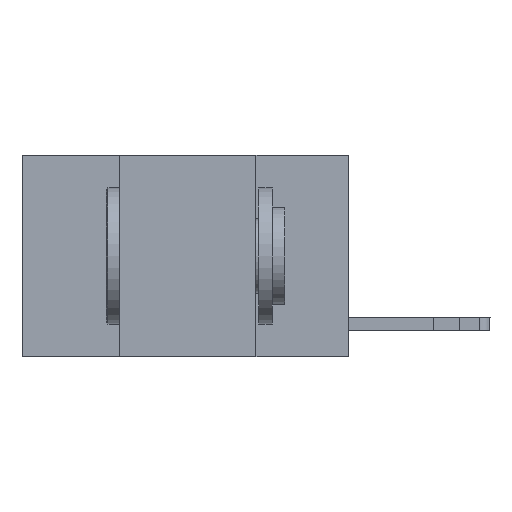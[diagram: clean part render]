
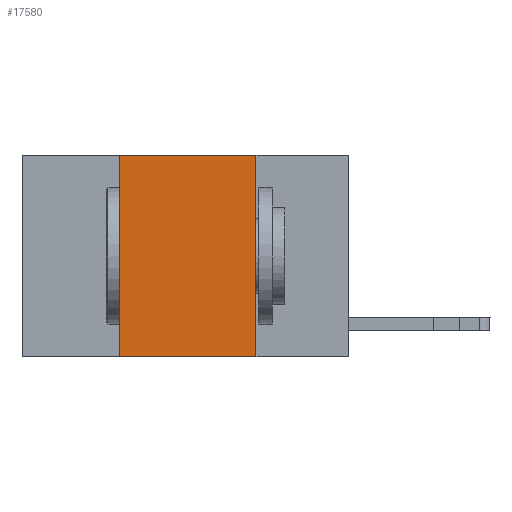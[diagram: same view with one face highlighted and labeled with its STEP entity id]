
A CAD part, left-side view. The second image highlights one B-rep face of the part: STEP entity #17580.
In plain terms, the highlighted planar face has unit normal (-1, 0, 0).
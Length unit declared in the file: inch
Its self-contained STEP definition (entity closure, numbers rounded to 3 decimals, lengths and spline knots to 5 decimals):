
#30 = VECTOR ( 'NONE', #4985, 39.37008 ) ;
#475 = EDGE_CURVE ( 'NONE', #6820, #13856, #2830, .T. ) ;
#1636 = ORIENTED_EDGE ( 'NONE', *, *, #10751, .F. ) ;
#2438 = LINE ( 'NONE', #6484, #4378 ) ;
#2540 = DIRECTION ( 'NONE',  ( 0., 0., -1. ) ) ;
#2546 = VERTEX_POINT ( 'NONE', #12381 ) ;
#2667 = VECTOR ( 'NONE', #17746, 39.37008 ) ;
#2830 = LINE ( 'NONE', #18895, #2667 ) ;
#3258 = EDGE_CURVE ( 'NONE', #6820, #6884, #4896, .T. ) ;
#3548 = CARTESIAN_POINT ( 'NONE',  ( 0., 0.6, -0.37 ) ) ;
#4378 = VECTOR ( 'NONE', #13952, 39.37008 ) ;
#4896 = LINE ( 'NONE', #3548, #30 ) ;
#4985 = DIRECTION ( 'NONE',  ( 0., -1., 0. ) ) ;
#5705 = EDGE_LOOP ( 'NONE', ( #7801, #1636, #15450, #14165 ) ) ;
#6484 = CARTESIAN_POINT ( 'NONE',  ( 0., 0.6, 0. ) ) ;
#6820 = VERTEX_POINT ( 'NONE', #11185 ) ;
#6884 = VERTEX_POINT ( 'NONE', #8869 ) ;
#7768 = DIRECTION ( 'NONE',  ( 1., 0., 0. ) ) ;
#7801 = ORIENTED_EDGE ( 'NONE', *, *, #15721, .F. ) ;
#8869 = CARTESIAN_POINT ( 'NONE',  ( 0., 0.17, -0.37 ) ) ;
#9119 = FACE_OUTER_BOUND ( 'NONE', #5705, .T. ) ;
#9667 = AXIS2_PLACEMENT_3D ( 'NONE', #18066, #7768, #10446 ) ;
#10446 = DIRECTION ( 'NONE',  ( 0., 0., -1. ) ) ;
#10751 = EDGE_CURVE ( 'NONE', #13856, #2546, #2438, .T. ) ;
#11185 = CARTESIAN_POINT ( 'NONE',  ( 0., 0.42, -0.37 ) ) ;
#12381 = CARTESIAN_POINT ( 'NONE',  ( 0., 0.17, 0. ) ) ;
#13856 = VERTEX_POINT ( 'NONE', #18139 ) ;
#13952 = DIRECTION ( 'NONE',  ( 0., -1., 0. ) ) ;
#14165 = ORIENTED_EDGE ( 'NONE', *, *, #3258, .T. ) ;
#14357 = LINE ( 'NONE', #15995, #17373 ) ;
#14789 = PLANE ( 'NONE',  #9667 ) ;
#15450 = ORIENTED_EDGE ( 'NONE', *, *, #475, .F. ) ;
#15721 = EDGE_CURVE ( 'NONE', #2546, #6884, #14357, .T. ) ;
#15995 = CARTESIAN_POINT ( 'NONE',  ( 0., 0.17, 0. ) ) ;
#17373 = VECTOR ( 'NONE', #2540, 39.37008 ) ;
#17580 = ADVANCED_FACE ( 'NONE', ( #9119 ), #14789, .F. ) ;
#17746 = DIRECTION ( 'NONE',  ( 0., 0., 1. ) ) ;
#18066 = CARTESIAN_POINT ( 'NONE',  ( 0., 0.6, 0. ) ) ;
#18139 = CARTESIAN_POINT ( 'NONE',  ( 0., 0.42, 0. ) ) ;
#18895 = CARTESIAN_POINT ( 'NONE',  ( 0., 0.42, 0. ) ) ;
